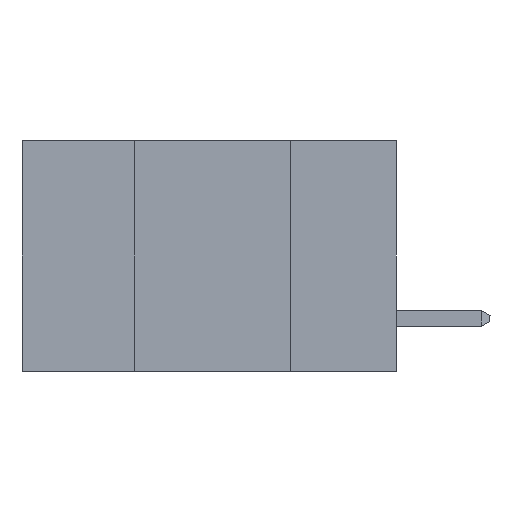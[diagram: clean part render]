
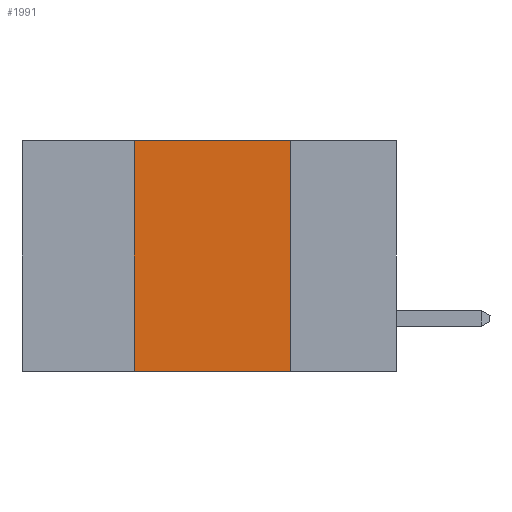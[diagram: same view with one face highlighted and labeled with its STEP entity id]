
A CAD part, left-side view. The second image highlights one B-rep face of the part: STEP entity #1991.
In plain terms, the highlighted planar face has unit normal (-1, 0, 0).
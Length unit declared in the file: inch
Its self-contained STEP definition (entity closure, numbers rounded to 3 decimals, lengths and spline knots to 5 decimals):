
#720 = CARTESIAN_POINT ( 'NONE',  ( 0., 0.17, 0. ) ) ;
#1991 = ADVANCED_FACE ( 'NONE', ( #19977 ), #2380, .F. ) ;
#2258 = CARTESIAN_POINT ( 'NONE',  ( 0., 0.17, -0.37 ) ) ;
#2380 = PLANE ( 'NONE',  #15931 ) ;
#2538 = CARTESIAN_POINT ( 'NONE',  ( 0., 0.6, 0. ) ) ;
#2797 = LINE ( 'NONE', #2885, #23387 ) ;
#2885 = CARTESIAN_POINT ( 'NONE',  ( 0., 0.6, -0.37 ) ) ;
#2890 = VERTEX_POINT ( 'NONE', #18035 ) ;
#4368 = EDGE_CURVE ( 'NONE', #9753, #2890, #2797, .T. ) ;
#4619 = ORIENTED_EDGE ( 'NONE', *, *, #9683, .F. ) ;
#5214 = EDGE_LOOP ( 'NONE', ( #25708, #4619, #15532, #14724 ) ) ;
#8273 = CARTESIAN_POINT ( 'NONE',  ( 0., 0.6, 0. ) ) ;
#9683 = EDGE_CURVE ( 'NONE', #17944, #15324, #14180, .T. ) ;
#9753 = VERTEX_POINT ( 'NONE', #18441 ) ;
#11732 = EDGE_CURVE ( 'NONE', #15324, #2890, #18718, .T. ) ;
#12288 = DIRECTION ( 'NONE',  ( 0., -1., 0. ) ) ;
#14145 = VECTOR ( 'NONE', #19268, 39.37008 ) ;
#14180 = LINE ( 'NONE', #8273, #24158 ) ;
#14724 = ORIENTED_EDGE ( 'NONE', *, *, #4368, .T. ) ;
#15324 = VERTEX_POINT ( 'NONE', #720 ) ;
#15532 = ORIENTED_EDGE ( 'NONE', *, *, #16661, .F. ) ;
#15931 = AXIS2_PLACEMENT_3D ( 'NONE', #2538, #16533, #20984 ) ;
#16533 = DIRECTION ( 'NONE',  ( 1., 0., 0. ) ) ;
#16661 = EDGE_CURVE ( 'NONE', #9753, #17944, #19455, .T. ) ;
#17272 = CARTESIAN_POINT ( 'NONE',  ( 0., 0.42, -0.37 ) ) ;
#17944 = VERTEX_POINT ( 'NONE', #21944 ) ;
#18035 = CARTESIAN_POINT ( 'NONE',  ( 0., 0.17, -0.37 ) ) ;
#18210 = DIRECTION ( 'NONE',  ( 0., 0., -1. ) ) ;
#18441 = CARTESIAN_POINT ( 'NONE',  ( 0., 0.42, -0.37 ) ) ;
#18718 = LINE ( 'NONE', #2258, #23408 ) ;
#18810 = DIRECTION ( 'NONE',  ( 0., -1., 0. ) ) ;
#19268 = DIRECTION ( 'NONE',  ( 0., 0., 1. ) ) ;
#19455 = LINE ( 'NONE', #17272, #14145 ) ;
#19977 = FACE_OUTER_BOUND ( 'NONE', #5214, .T. ) ;
#20984 = DIRECTION ( 'NONE',  ( 0., 0., -1. ) ) ;
#21944 = CARTESIAN_POINT ( 'NONE',  ( 0., 0.42, 0. ) ) ;
#23387 = VECTOR ( 'NONE', #18810, 39.37008 ) ;
#23408 = VECTOR ( 'NONE', #18210, 39.37008 ) ;
#24158 = VECTOR ( 'NONE', #12288, 39.37008 ) ;
#25708 = ORIENTED_EDGE ( 'NONE', *, *, #11732, .F. ) ;
